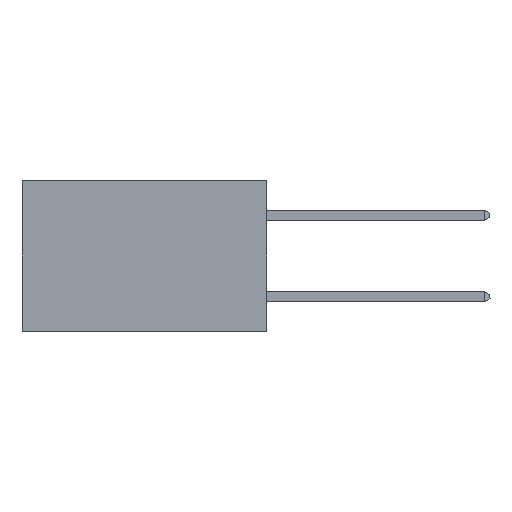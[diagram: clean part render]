
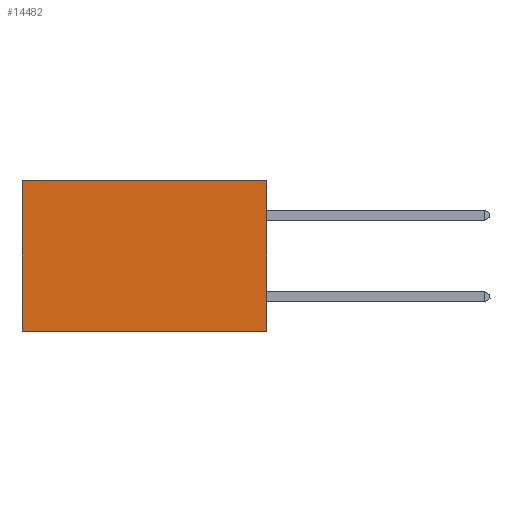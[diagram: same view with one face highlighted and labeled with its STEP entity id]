
A CAD part, left-side view. The second image highlights one B-rep face of the part: STEP entity #14482.
In plain terms, the highlighted planar face has unit normal (-1, 0, 0).
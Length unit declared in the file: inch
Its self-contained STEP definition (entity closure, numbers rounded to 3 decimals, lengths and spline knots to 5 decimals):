
#39 = CARTESIAN_POINT ( 'NONE',  ( 0.2875, 0.6, 0. ) ) ;
#192 = DIRECTION ( 'NONE',  ( 0., 0., -1. ) ) ;
#195 = VERTEX_POINT ( 'NONE', #8943 ) ;
#834 = VECTOR ( 'NONE', #192, 39.37008 ) ;
#973 = CARTESIAN_POINT ( 'NONE',  ( 0.2875, 0., -0.37 ) ) ;
#1772 = CARTESIAN_POINT ( 'NONE',  ( 0.2875, 0., -0.37 ) ) ;
#1878 = VERTEX_POINT ( 'NONE', #973 ) ;
#1882 = DIRECTION ( 'NONE',  ( 0., 1., 0. ) ) ;
#2233 = CARTESIAN_POINT ( 'NONE',  ( 0.2875, 0., 0. ) ) ;
#2572 = ORIENTED_EDGE ( 'NONE', *, *, #2651, .F. ) ;
#2651 = EDGE_CURVE ( 'NONE', #1878, #195, #11657, .T. ) ;
#3950 = LINE ( 'NONE', #39, #834 ) ;
#4270 = AXIS2_PLACEMENT_3D ( 'NONE', #8938, #6497, #10079 ) ;
#4486 = VECTOR ( 'NONE', #1882, 39.37008 ) ;
#6077 = EDGE_CURVE ( 'NONE', #13420, #12153, #12579, .T. ) ;
#6191 = EDGE_CURVE ( 'NONE', #12153, #195, #3950, .T. ) ;
#6497 = DIRECTION ( 'NONE',  ( 1., 0., 0. ) ) ;
#7856 = CARTESIAN_POINT ( 'NONE',  ( 0.2875, 0., 0. ) ) ;
#7880 = VECTOR ( 'NONE', #9178, 39.37008 ) ;
#8206 = ORIENTED_EDGE ( 'NONE', *, *, #6077, .T. ) ;
#8938 = CARTESIAN_POINT ( 'NONE',  ( 0.2875, 0., 0. ) ) ;
#8943 = CARTESIAN_POINT ( 'NONE',  ( 0.2875, 0.6, -0.37 ) ) ;
#9016 = CARTESIAN_POINT ( 'NONE',  ( 0.2875, 0.6, 0. ) ) ;
#9045 = FACE_OUTER_BOUND ( 'NONE', #14825, .T. ) ;
#9178 = DIRECTION ( 'NONE',  ( 0., 0., -1. ) ) ;
#9684 = EDGE_CURVE ( 'NONE', #13420, #1878, #13028, .T. ) ;
#10079 = DIRECTION ( 'NONE',  ( 0., 0., -1. ) ) ;
#10965 = CARTESIAN_POINT ( 'NONE',  ( 0.2875, 0., 0. ) ) ;
#11156 = ORIENTED_EDGE ( 'NONE', *, *, #9684, .F. ) ;
#11657 = LINE ( 'NONE', #1772, #4486 ) ;
#11667 = VECTOR ( 'NONE', #12159, 39.37008 ) ;
#12153 = VERTEX_POINT ( 'NONE', #9016 ) ;
#12159 = DIRECTION ( 'NONE',  ( 0., 1., 0. ) ) ;
#12579 = LINE ( 'NONE', #10965, #11667 ) ;
#12956 = ORIENTED_EDGE ( 'NONE', *, *, #6191, .T. ) ;
#13028 = LINE ( 'NONE', #2233, #7880 ) ;
#13420 = VERTEX_POINT ( 'NONE', #7856 ) ;
#14482 = ADVANCED_FACE ( 'NONE', ( #9045 ), #14604, .F. ) ;
#14604 = PLANE ( 'NONE',  #4270 ) ;
#14825 = EDGE_LOOP ( 'NONE', ( #12956, #2572, #11156, #8206 ) ) ;
